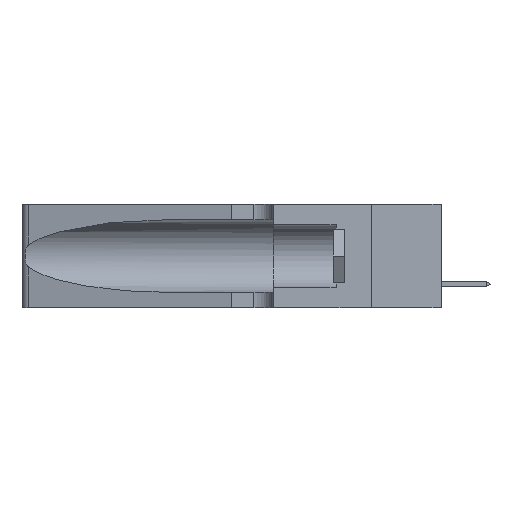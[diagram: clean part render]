
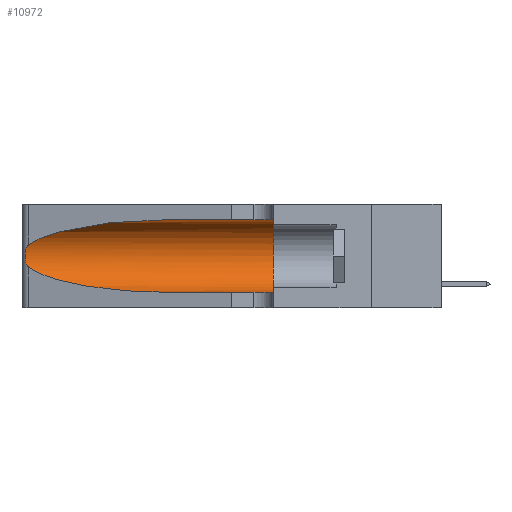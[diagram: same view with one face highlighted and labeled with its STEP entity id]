
A CAD part, left-side view. The second image highlights one B-rep face of the part: STEP entity #10972.
In plain terms, the highlighted cylindrical face has radius 3.308 mm (diameter 6.617 mm), a partial arc.
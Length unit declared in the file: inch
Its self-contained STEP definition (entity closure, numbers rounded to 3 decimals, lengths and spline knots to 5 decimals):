
#517 = AXIS2_PLACEMENT_3D ( 'NONE', #18959, #15214, #7040 ) ;
#963 = CARTESIAN_POINT ( 'NONE',  ( 0.25854, 1.2359, 0.20912 ) ) ;
#1059 = CARTESIAN_POINT ( 'NONE',  ( 0.26017, 1.23833, 0.17102 ) ) ;
#1418 = LINE ( 'NONE', #18325, #13971 ) ;
#2935 =( BOUNDED_CURVE ( )  B_SPLINE_CURVE ( 3, ( #12553, #14685, #5770, #21439 ),
 .UNSPECIFIED., .F., .T. ) 
 B_SPLINE_CURVE_WITH_KNOTS ( ( 4, 4 ),
 ( 3.44316, 4.71239 ),
 .UNSPECIFIED. ) 
 CURVE ( )  GEOMETRIC_REPRESENTATION_ITEM ( )  RATIONAL_B_SPLINE_CURVE ( ( 1., 0.87, 0.87, 1. ) ) 
 REPRESENTATION_ITEM ( '' )  );
#4607 = CARTESIAN_POINT ( 'NONE',  ( 0.18966, 0.96281, 0.31525 ) ) ;
#4780 = CARTESIAN_POINT ( 'NONE',  ( 0.25639, 1.23186, 0.15144 ) ) ;
#4873 = CARTESIAN_POINT ( 'NONE',  ( 0.25789, 1.23486, 0.15765 ) ) ;
#5770 = CARTESIAN_POINT ( 'NONE',  ( 0.18966, 0.96281, 0.05475 ) ) ;
#6824 = VERTEX_POINT ( 'NONE', #23281 ) ;
#7035 = CARTESIAN_POINT ( 'NONE',  ( 0.25487, 1.22718, 0.14631 ) ) ;
#7040 = DIRECTION ( 'NONE',  ( 0., 0., -1. ) ) ;
#7089 = CARTESIAN_POINT ( 'NONE',  ( 0.25856, 1.23593, 0.16098 ) ) ;
#8177 = EDGE_CURVE ( 'NONE', #28363, #24549, #1418, .T. ) ;
#9207 = EDGE_CURVE ( 'NONE', #10321, #24549, #14610, .T. ) ;
#9238 = DIRECTION ( 'NONE',  ( 0., 0., 1. ) ) ;
#9856 = ORIENTED_EDGE ( 'NONE', *, *, #8177, .T. ) ;
#9952 = CARTESIAN_POINT ( 'NONE',  ( 0.26075, 1.23896, 0.19203 ) ) ;
#10000 = LINE ( 'NONE', #12502, #11751 ) ;
#10297 = B_SPLINE_CURVE_WITH_KNOTS ( 'NONE', 3,
 ( #21302, #20494, #21101, #25478, #963, #24965, #9952, #14441, #1059, #7089, #4873, #4780, #22592, #7035 ),
 .UNSPECIFIED., .F., .F.,
 ( 4, 2, 2, 2, 2, 2, 4 ),
 ( 0., 0.00027, 0.00053, 0.00107, 0.0016, 0.00187, 0.00214 ),
 .UNSPECIFIED. ) ;
#10321 = VERTEX_POINT ( 'NONE', #15873 ) ;
#10972 = ADVANCED_FACE ( 'NONE', ( #11686 ), #12020, .F. ) ;
#11370 = CARTESIAN_POINT ( 'NONE',  ( 0.2373, 1.15595, 0.28018 ) ) ;
#11686 = FACE_OUTER_BOUND ( 'NONE', #19916, .T. ) ;
#11751 = VECTOR ( 'NONE', #16697, 39.37008 ) ;
#12020 = CYLINDRICAL_SURFACE ( 'NONE', #517, 0.13025 ) ;
#12111 = CARTESIAN_POINT ( 'NONE',  ( 0.25487, 1.22718, 0.14631 ) ) ;
#12502 = CARTESIAN_POINT ( 'NONE',  ( 0.1305, 1.61858, 0.31525 ) ) ;
#12553 = CARTESIAN_POINT ( 'NONE',  ( 0.25487, 1.22718, 0.14631 ) ) ;
#13322 = CARTESIAN_POINT ( 'NONE',  ( 0.1305, 0.72297, 0.31525 ) ) ;
#13971 = VECTOR ( 'NONE', #27466, 39.37008 ) ;
#14441 = CARTESIAN_POINT ( 'NONE',  ( 0.26075, 1.23896, 0.178 ) ) ;
#14610 = CIRCLE ( 'NONE', #23520, 0.13025 ) ;
#14685 = CARTESIAN_POINT ( 'NONE',  ( 0.2373, 1.15595, 0.08982 ) ) ;
#15045 = EDGE_CURVE ( 'NONE', #21339, #25642, #10297, .T. ) ;
#15214 = DIRECTION ( 'NONE',  ( 0., -1., 0. ) ) ;
#15873 = CARTESIAN_POINT ( 'NONE',  ( 0.1305, 0.35, 0.31525 ) ) ;
#16068 = DIRECTION ( 'NONE',  ( 0., 1., 0. ) ) ;
#16697 = DIRECTION ( 'NONE',  ( 0., -1., 0. ) ) ;
#16876 = ORIENTED_EDGE ( 'NONE', *, *, #18505, .T. ) ;
#16886 = CARTESIAN_POINT ( 'NONE',  ( 0.1305, 0.72297, 0.05475 ) ) ;
#18325 = CARTESIAN_POINT ( 'NONE',  ( 0.1305, 1.61858, 0.05475 ) ) ;
#18505 = EDGE_CURVE ( 'NONE', #6824, #21339, #26378, .T. ) ;
#18676 = ORIENTED_EDGE ( 'NONE', *, *, #15045, .T. ) ;
#18959 = CARTESIAN_POINT ( 'NONE',  ( 0.1305, 1.61858, 0.185 ) ) ;
#19916 = EDGE_LOOP ( 'NONE', ( #16876, #18676, #26831, #9856, #21807, #25216 ) ) ;
#20494 = CARTESIAN_POINT ( 'NONE',  ( 0.25555, 1.22994, 0.2215 ) ) ;
#21101 = CARTESIAN_POINT ( 'NONE',  ( 0.25639, 1.23184, 0.21858 ) ) ;
#21302 = CARTESIAN_POINT ( 'NONE',  ( 0.25487, 1.22718, 0.22369 ) ) ;
#21339 = VERTEX_POINT ( 'NONE', #28227 ) ;
#21439 = CARTESIAN_POINT ( 'NONE',  ( 0.1305, 0.72297, 0.05475 ) ) ;
#21807 = ORIENTED_EDGE ( 'NONE', *, *, #9207, .F. ) ;
#22592 = CARTESIAN_POINT ( 'NONE',  ( 0.25555, 1.22993, 0.14849 ) ) ;
#23195 = EDGE_CURVE ( 'NONE', #6824, #10321, #10000, .T. ) ;
#23281 = CARTESIAN_POINT ( 'NONE',  ( 0.1305, 0.72297, 0.31525 ) ) ;
#23316 = CARTESIAN_POINT ( 'NONE',  ( 0.1305, 0.35, 0.05475 ) ) ;
#23520 = AXIS2_PLACEMENT_3D ( 'NONE', #26535, #16068, #9238 ) ;
#24549 = VERTEX_POINT ( 'NONE', #23316 ) ;
#24965 = CARTESIAN_POINT ( 'NONE',  ( 0.26018, 1.23835, 0.19895 ) ) ;
#25216 = ORIENTED_EDGE ( 'NONE', *, *, #23195, .F. ) ;
#25478 = CARTESIAN_POINT ( 'NONE',  ( 0.25787, 1.23484, 0.2124 ) ) ;
#25642 = VERTEX_POINT ( 'NONE', #12111 ) ;
#26378 =( BOUNDED_CURVE ( )  B_SPLINE_CURVE ( 3, ( #13322, #4607, #11370, #26591 ),
 .UNSPECIFIED., .F., .F. ) 
 B_SPLINE_CURVE_WITH_KNOTS ( ( 4, 4 ),
 ( 1.5708, 2.84003 ),
 .UNSPECIFIED. ) 
 CURVE ( )  GEOMETRIC_REPRESENTATION_ITEM ( )  RATIONAL_B_SPLINE_CURVE ( ( 1., 0.87, 0.87, 1. ) ) 
 REPRESENTATION_ITEM ( '' )  );
#26535 = CARTESIAN_POINT ( 'NONE',  ( 0.1305, 0.35, 0.185 ) ) ;
#26591 = CARTESIAN_POINT ( 'NONE',  ( 0.25487, 1.22718, 0.22369 ) ) ;
#26831 = ORIENTED_EDGE ( 'NONE', *, *, #27229, .T. ) ;
#27229 = EDGE_CURVE ( 'NONE', #25642, #28363, #2935, .T. ) ;
#27466 = DIRECTION ( 'NONE',  ( 0., -1., 0. ) ) ;
#28227 = CARTESIAN_POINT ( 'NONE',  ( 0.25487, 1.22718, 0.22369 ) ) ;
#28363 = VERTEX_POINT ( 'NONE', #16886 ) ;
